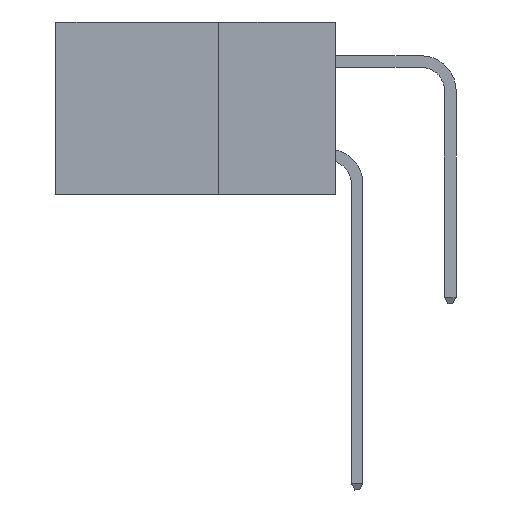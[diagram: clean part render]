
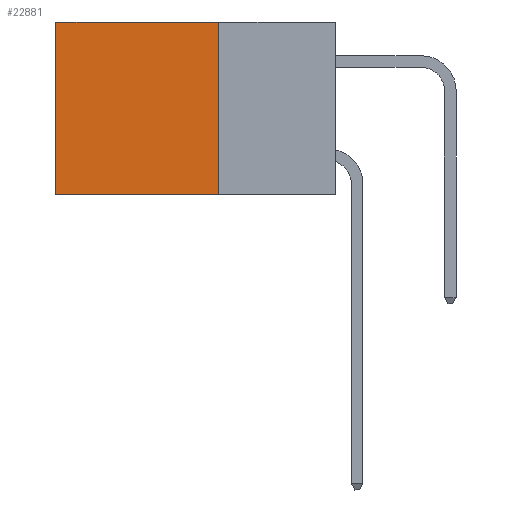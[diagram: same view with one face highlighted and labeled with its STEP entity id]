
A CAD part, left-side view. The second image highlights one B-rep face of the part: STEP entity #22881.
In plain terms, the highlighted planar face has unit normal (-1, 0, 0).
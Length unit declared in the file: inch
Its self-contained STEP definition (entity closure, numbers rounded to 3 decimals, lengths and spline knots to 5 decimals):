
#519 = CARTESIAN_POINT ( 'NONE',  ( 0.2875, 0.25, 0. ) ) ;
#1844 = CARTESIAN_POINT ( 'NONE',  ( 0.2875, 0.6, 0. ) ) ;
#2146 = LINE ( 'NONE', #24813, #23501 ) ;
#3546 = EDGE_CURVE ( 'NONE', #5760, #11438, #2146, .T. ) ;
#3750 = ORIENTED_EDGE ( 'NONE', *, *, #17097, .T. ) ;
#4364 = EDGE_LOOP ( 'NONE', ( #22869, #11995, #7743, #3750 ) ) ;
#5151 = CARTESIAN_POINT ( 'NONE',  ( 0.2875, 0.25, -0.37 ) ) ;
#5285 = CARTESIAN_POINT ( 'NONE',  ( 0.2875, 0.6, -0.37 ) ) ;
#5760 = VERTEX_POINT ( 'NONE', #10508 ) ;
#6011 = EDGE_CURVE ( 'NONE', #14074, #12449, #9231, .T. ) ;
#6754 = CARTESIAN_POINT ( 'NONE',  ( 0.2875, 0.25, -0.37 ) ) ;
#7429 = VECTOR ( 'NONE', #9745, 39.37008 ) ;
#7743 = ORIENTED_EDGE ( 'NONE', *, *, #3546, .F. ) ;
#8898 = DIRECTION ( 'NONE',  ( 0., 0., -1. ) ) ;
#9058 = DIRECTION ( 'NONE',  ( 1., 0., 0. ) ) ;
#9231 = LINE ( 'NONE', #1844, #7429 ) ;
#9402 = DIRECTION ( 'NONE',  ( 0., 0., -1. ) ) ;
#9420 = AXIS2_PLACEMENT_3D ( 'NONE', #10813, #9058, #8898 ) ;
#9745 = DIRECTION ( 'NONE',  ( 0., 0., -1. ) ) ;
#10508 = CARTESIAN_POINT ( 'NONE',  ( 0.2875, 0.25, 0. ) ) ;
#10698 = DIRECTION ( 'NONE',  ( 0., 1., 0. ) ) ;
#10813 = CARTESIAN_POINT ( 'NONE',  ( 0.2875, 0.25, 0. ) ) ;
#11438 = VERTEX_POINT ( 'NONE', #5151 ) ;
#11547 = EDGE_CURVE ( 'NONE', #11438, #12449, #14113, .T. ) ;
#11995 = ORIENTED_EDGE ( 'NONE', *, *, #11547, .F. ) ;
#12301 = CARTESIAN_POINT ( 'NONE',  ( 0.2875, 0.6, 0. ) ) ;
#12449 = VERTEX_POINT ( 'NONE', #5285 ) ;
#13188 = LINE ( 'NONE', #519, #20369 ) ;
#14074 = VERTEX_POINT ( 'NONE', #12301 ) ;
#14113 = LINE ( 'NONE', #6754, #18279 ) ;
#16035 = DIRECTION ( 'NONE',  ( 0., 1., 0. ) ) ;
#17097 = EDGE_CURVE ( 'NONE', #5760, #14074, #13188, .T. ) ;
#18279 = VECTOR ( 'NONE', #10698, 39.37008 ) ;
#20369 = VECTOR ( 'NONE', #16035, 39.37008 ) ;
#20541 = PLANE ( 'NONE',  #9420 ) ;
#20977 = FACE_OUTER_BOUND ( 'NONE', #4364, .T. ) ;
#22869 = ORIENTED_EDGE ( 'NONE', *, *, #6011, .T. ) ;
#22881 = ADVANCED_FACE ( 'NONE', ( #20977 ), #20541, .F. ) ;
#23501 = VECTOR ( 'NONE', #9402, 39.37008 ) ;
#24813 = CARTESIAN_POINT ( 'NONE',  ( 0.2875, 0.25, 0. ) ) ;
